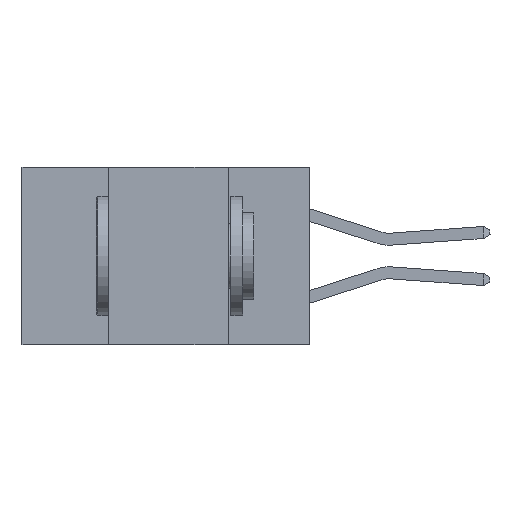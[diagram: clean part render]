
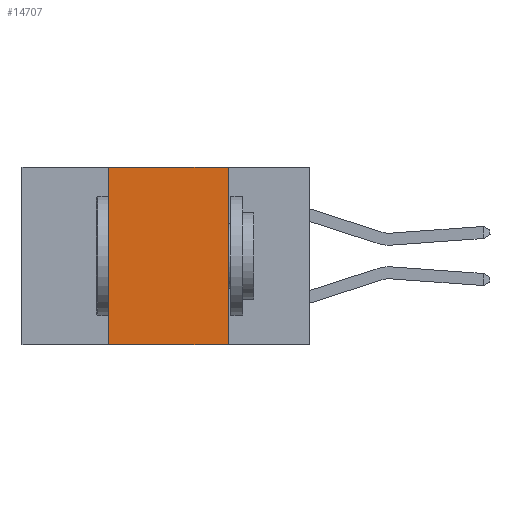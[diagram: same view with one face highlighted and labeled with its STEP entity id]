
A CAD part, left-side view. The second image highlights one B-rep face of the part: STEP entity #14707.
In plain terms, the highlighted planar face has unit normal (-1, 0, 0).
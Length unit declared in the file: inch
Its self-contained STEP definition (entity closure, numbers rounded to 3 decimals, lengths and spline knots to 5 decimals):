
#760 = CARTESIAN_POINT ( 'NONE',  ( 0., 0.17, -0.37 ) ) ;
#902 = VERTEX_POINT ( 'NONE', #7541 ) ;
#938 = EDGE_CURVE ( 'NONE', #26062, #902, #2453, .T. ) ;
#1558 = LINE ( 'NONE', #12133, #21915 ) ;
#2453 = LINE ( 'NONE', #16826, #8511 ) ;
#3182 = CARTESIAN_POINT ( 'NONE',  ( 0., 0.6, -0.37 ) ) ;
#5822 = VECTOR ( 'NONE', #14641, 39.37008 ) ;
#5993 = ORIENTED_EDGE ( 'NONE', *, *, #938, .F. ) ;
#7229 = VERTEX_POINT ( 'NONE', #760 ) ;
#7541 = CARTESIAN_POINT ( 'NONE',  ( 0., 0.17, 0. ) ) ;
#7789 = EDGE_CURVE ( 'NONE', #902, #7229, #10534, .T. ) ;
#8219 = DIRECTION ( 'NONE',  ( 0., 0., -1. ) ) ;
#8511 = VECTOR ( 'NONE', #11229, 39.37008 ) ;
#10531 = CARTESIAN_POINT ( 'NONE',  ( 0., 0.17, 0. ) ) ;
#10534 = LINE ( 'NONE', #10531, #5822 ) ;
#10867 = CARTESIAN_POINT ( 'NONE',  ( 0., 0.42, -0.37 ) ) ;
#11229 = DIRECTION ( 'NONE',  ( 0., -1., 0. ) ) ;
#11801 = FACE_OUTER_BOUND ( 'NONE', #21149, .T. ) ;
#12133 = CARTESIAN_POINT ( 'NONE',  ( 0., 0.42, 0. ) ) ;
#14074 = CARTESIAN_POINT ( 'NONE',  ( 0., 0.6, 0. ) ) ;
#14244 = PLANE ( 'NONE',  #23084 ) ;
#14261 = VERTEX_POINT ( 'NONE', #10867 ) ;
#14641 = DIRECTION ( 'NONE',  ( 0., 0., -1. ) ) ;
#14707 = ADVANCED_FACE ( 'NONE', ( #11801 ), #14244, .F. ) ;
#14909 = LINE ( 'NONE', #3182, #20320 ) ;
#15267 = CARTESIAN_POINT ( 'NONE',  ( 0., 0.42, 0. ) ) ;
#16826 = CARTESIAN_POINT ( 'NONE',  ( 0., 0.6, 0. ) ) ;
#18282 = DIRECTION ( 'NONE',  ( 0., 0., 1. ) ) ;
#19434 = DIRECTION ( 'NONE',  ( 0., -1., 0. ) ) ;
#20320 = VECTOR ( 'NONE', #19434, 39.37008 ) ;
#20382 = DIRECTION ( 'NONE',  ( 1., 0., 0. ) ) ;
#20825 = EDGE_CURVE ( 'NONE', #14261, #26062, #1558, .T. ) ;
#21149 = EDGE_LOOP ( 'NONE', ( #24375, #5993, #21540, #22799 ) ) ;
#21540 = ORIENTED_EDGE ( 'NONE', *, *, #20825, .F. ) ;
#21915 = VECTOR ( 'NONE', #18282, 39.37008 ) ;
#22799 = ORIENTED_EDGE ( 'NONE', *, *, #25050, .T. ) ;
#23084 = AXIS2_PLACEMENT_3D ( 'NONE', #14074, #20382, #8219 ) ;
#24375 = ORIENTED_EDGE ( 'NONE', *, *, #7789, .F. ) ;
#25050 = EDGE_CURVE ( 'NONE', #14261, #7229, #14909, .T. ) ;
#26062 = VERTEX_POINT ( 'NONE', #15267 ) ;
